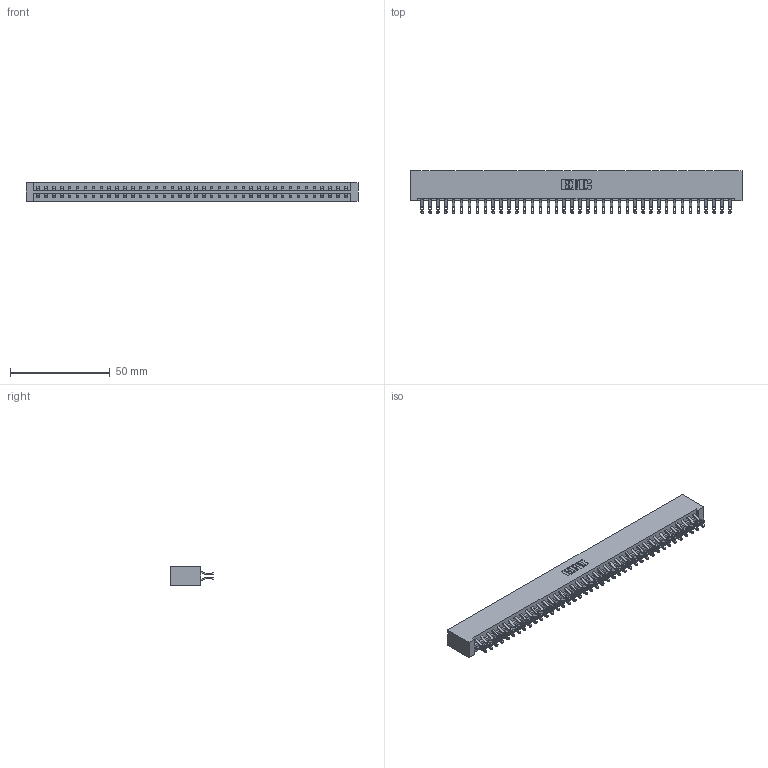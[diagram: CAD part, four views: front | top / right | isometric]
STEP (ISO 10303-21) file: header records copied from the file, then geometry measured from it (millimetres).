
FILE_DESCRIPTION (( 'STEP AP203' ), '1' );
FILE_NAME ('833-080-555-201.STEP', '2020-06-05T22:12:59', ( '' ), ( '' ), 'SwSTEP 2.0', 'SolidWorks 2020', '' );
FILE_SCHEMA (( 'CONFIG_CONTROL_DESIGN' ));
Length unit declared in the file: inch
Products named in the file (3): 833-080-555-201; 345-292-001_555 Tail; 833 Part_Lugless
Assembly tree (81 placements, depth 2):
  833-080-555-201
    833 Part_Lugless
    345-292-001_555 Tail  x80
Bounding box: 166.75 x 21.47 x 9.4 mm (x, y, z)
Volume: 17869.9 mm3; surface area: 21997.3 mm2
Topology: 81 solids, 81 shells, 4746 faces, 14927 edges, 9950 vertices
Faces by surface type: plane 2786, cylinder 1960
Entity records: 26041 total; most frequent: CARTESIAN_POINT 4352, ORIENTED_EDGE 4258, DIRECTION 3685, EDGE_CURVE 2129, VECTOR 1989, LINE 1989, VERTEX_POINT 1418, AXIS2_PLACEMENT_3D 848
